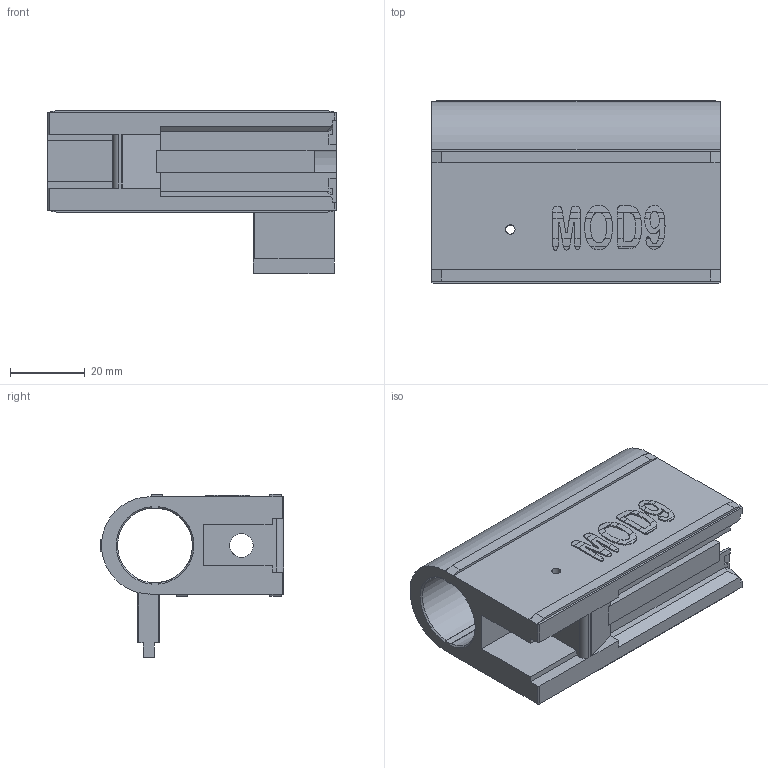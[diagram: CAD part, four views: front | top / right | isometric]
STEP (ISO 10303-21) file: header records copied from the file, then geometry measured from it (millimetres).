
FILE_DESCRIPTION(('STEP AP214'),'1');
FILE_NAME('Mod9 Bolt Carrier Final.stp','2020-09-28T22:41:55',(' '),(' '),'Spatial InterOp 3D',' ',' ');
FILE_SCHEMA(('AUTOMOTIVE_DESIGN { 1 0 10303 214 1 1 1 1 }'));
Length unit declared in the file: metre
Products named in the file (1): ASM Body
Bounding box: 77.19 x 48.98 x 43.65 mm (x, y, z)
Volume: 45920.7 mm3; surface area: 22156.7 mm2
Topology: 1 solids, 1 shells, 304 faces, 884 edges, 584 vertices
Faces by surface type: plane 142, bspline 125, cylinder 35, cone 2
Entity records: 12061 total; most frequent: CARTESIAN_POINT 4835, ORIENTED_EDGE 1768, DIRECTION 1067, EDGE_CURVE 884, VERTEX_POINT 584, LINE 519, VECTOR 519, EDGE_LOOP 314
